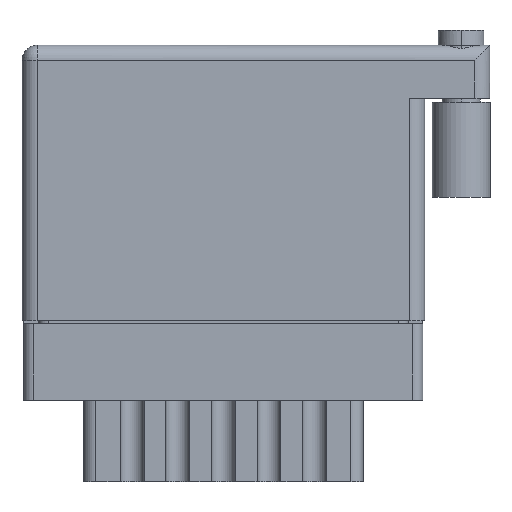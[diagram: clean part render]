
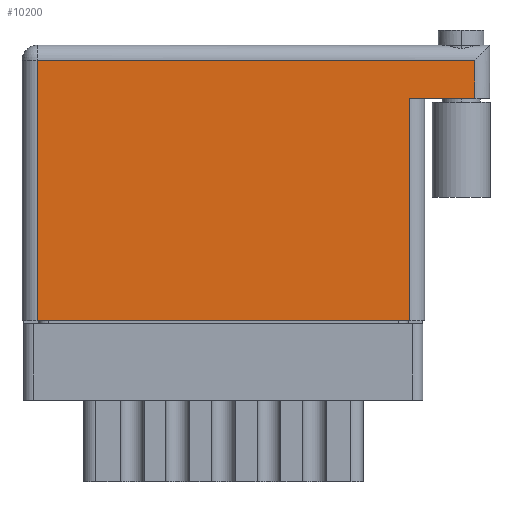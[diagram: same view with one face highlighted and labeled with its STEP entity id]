
A CAD part, front view. The second image highlights one B-rep face of the part: STEP entity #10200.
In plain terms, the highlighted face is planar.
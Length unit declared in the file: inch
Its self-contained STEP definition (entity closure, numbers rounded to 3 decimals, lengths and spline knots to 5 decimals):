
#524 = CARTESIAN_POINT ( 'NONE',  ( 0.05, 0., 0. ) ) ;
#576 = AXIS2_PLACEMENT_3D ( 'NONE', #20076, #8582, #14406 ) ;
#2120 = FACE_OUTER_BOUND ( 'NONE', #24671, .T. ) ;
#2966 = CARTESIAN_POINT ( 'NONE',  ( 0., 0.856, 0. ) ) ;
#3097 = DIRECTION ( 'NONE',  ( 0., 1., 0. ) ) ;
#3180 = DIRECTION ( 'NONE',  ( 1., 0., 0. ) ) ;
#4686 = DIRECTION ( 'NONE',  ( -1., 0., 0. ) ) ;
#4888 = CARTESIAN_POINT ( 'NONE',  ( 0., 0., 0. ) ) ;
#5067 = CARTESIAN_POINT ( 'NONE',  ( 1.275, 0.731, 0. ) ) ;
#5499 = CARTESIAN_POINT ( 'NONE',  ( 0.05, 0.856, 0. ) ) ;
#6198 = EDGE_CURVE ( 'NONE', #20927, #14190, #10894, .T. ) ;
#6744 = ORIENTED_EDGE ( 'NONE', *, *, #9987, .T. ) ;
#7228 = LINE ( 'NONE', #10571, #17594 ) ;
#7770 = ORIENTED_EDGE ( 'NONE', *, *, #10291, .T. ) ;
#7940 = ORIENTED_EDGE ( 'NONE', *, *, #13124, .T. ) ;
#8337 = LINE ( 'NONE', #15864, #14814 ) ;
#8572 = VECTOR ( 'NONE', #3180, 39.37008 ) ;
#8582 = DIRECTION ( 'NONE',  ( 0., 0., -1. ) ) ;
#9447 = CARTESIAN_POINT ( 'NONE',  ( 1.275, 0.731, 0. ) ) ;
#9789 = ORIENTED_EDGE ( 'NONE', *, *, #19190, .F. ) ;
#9987 = EDGE_CURVE ( 'NONE', #21195, #25433, #21282, .T. ) ;
#10181 = DIRECTION ( 'NONE',  ( 0., -1., 0. ) ) ;
#10200 = ADVANCED_FACE ( 'NONE', ( #2120 ), #22199, .F. ) ;
#10291 = EDGE_CURVE ( 'NONE', #14190, #21195, #10573, .T. ) ;
#10571 = CARTESIAN_POINT ( 'NONE',  ( 1.539, 0.731, 0. ) ) ;
#10573 = LINE ( 'NONE', #524, #11986 ) ;
#10894 = LINE ( 'NONE', #2966, #17173 ) ;
#11986 = VECTOR ( 'NONE', #10181, 39.37008 ) ;
#13124 = EDGE_CURVE ( 'NONE', #21207, #20927, #8337, .T. ) ;
#14190 = VERTEX_POINT ( 'NONE', #5499 ) ;
#14406 = DIRECTION ( 'NONE',  ( -1., 0., 0. ) ) ;
#14814 = VECTOR ( 'NONE', #20367, 39.37008 ) ;
#15864 = CARTESIAN_POINT ( 'NONE',  ( 1.489, 0.906, 0. ) ) ;
#17173 = VECTOR ( 'NONE', #4686, 39.37008 ) ;
#17594 = VECTOR ( 'NONE', #20610, 39.37008 ) ;
#17921 = CARTESIAN_POINT ( 'NONE',  ( 1.489, 0.731, 0. ) ) ;
#19190 = EDGE_CURVE ( 'NONE', #21207, #22219, #7228, .T. ) ;
#19894 = ORIENTED_EDGE ( 'NONE', *, *, #25081, .T. ) ;
#20076 = CARTESIAN_POINT ( 'NONE',  ( 0., 0.906, 0. ) ) ;
#20170 = VECTOR ( 'NONE', #3097, 39.37008 ) ;
#20367 = DIRECTION ( 'NONE',  ( 0., 1., 0. ) ) ;
#20610 = DIRECTION ( 'NONE',  ( -1., 0., 0. ) ) ;
#20927 = VERTEX_POINT ( 'NONE', #21356 ) ;
#21195 = VERTEX_POINT ( 'NONE', #23856 ) ;
#21207 = VERTEX_POINT ( 'NONE', #17921 ) ;
#21282 = LINE ( 'NONE', #4888, #8572 ) ;
#21356 = CARTESIAN_POINT ( 'NONE',  ( 1.489, 0.856, 0. ) ) ;
#22096 = ORIENTED_EDGE ( 'NONE', *, *, #6198, .T. ) ;
#22199 = PLANE ( 'NONE',  #576 ) ;
#22219 = VERTEX_POINT ( 'NONE', #9447 ) ;
#23856 = CARTESIAN_POINT ( 'NONE',  ( 0.05, 0., 0. ) ) ;
#24666 = LINE ( 'NONE', #5067, #20170 ) ;
#24671 = EDGE_LOOP ( 'NONE', ( #6744, #19894, #9789, #7940, #22096, #7770 ) ) ;
#24984 = CARTESIAN_POINT ( 'NONE',  ( 1.275, 0., 0. ) ) ;
#25081 = EDGE_CURVE ( 'NONE', #25433, #22219, #24666, .T. ) ;
#25433 = VERTEX_POINT ( 'NONE', #24984 ) ;
